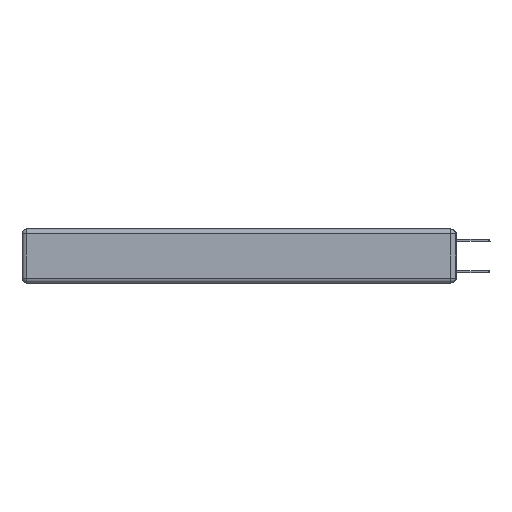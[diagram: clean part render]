
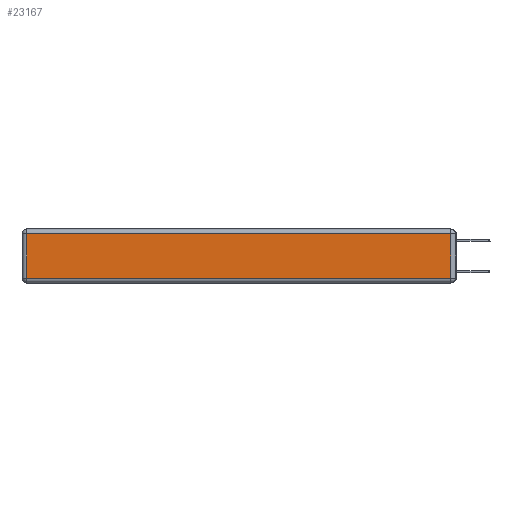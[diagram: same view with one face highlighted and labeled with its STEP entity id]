
A CAD part, left-side view. The second image highlights one B-rep face of the part: STEP entity #23167.
In plain terms, the highlighted planar face has unit normal (-1, 0, 0).
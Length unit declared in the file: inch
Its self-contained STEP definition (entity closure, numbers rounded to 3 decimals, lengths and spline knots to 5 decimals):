
#309 = DIRECTION ( 'NONE',  ( 0., 1., 0. ) ) ;
#857 = EDGE_CURVE ( 'NONE', #17902, #1594, #20052, .T. ) ;
#974 = CARTESIAN_POINT ( 'NONE',  ( 0., 2.72, -0.313 ) ) ;
#1301 = EDGE_CURVE ( 'NONE', #1594, #5061, #3868, .T. ) ;
#1594 = VERTEX_POINT ( 'NONE', #21425 ) ;
#1880 = ORIENTED_EDGE ( 'NONE', *, *, #857, .T. ) ;
#2568 = VECTOR ( 'NONE', #7059, 39.37008 ) ;
#2606 = VECTOR ( 'NONE', #11007, 39.37008 ) ;
#3868 = LINE ( 'NONE', #16387, #11226 ) ;
#5061 = VERTEX_POINT ( 'NONE', #16418 ) ;
#5471 = VECTOR ( 'NONE', #5655, 39.37008 ) ;
#5655 = DIRECTION ( 'NONE',  ( 0., -1., 0. ) ) ;
#7059 = DIRECTION ( 'NONE',  ( 0., 0., 1. ) ) ;
#7180 = CARTESIAN_POINT ( 'NONE',  ( 0., 0., -0.313 ) ) ;
#7407 = LINE ( 'NONE', #7180, #5471 ) ;
#8812 = ORIENTED_EDGE ( 'NONE', *, *, #8959, .T. ) ;
#8893 = LINE ( 'NONE', #9234, #2606 ) ;
#8959 = EDGE_CURVE ( 'NONE', #5061, #10770, #8893, .T. ) ;
#9234 = CARTESIAN_POINT ( 'NONE',  ( 0., 2.72, -0.343 ) ) ;
#9873 = EDGE_LOOP ( 'NONE', ( #12461, #1880, #17489, #8812 ) ) ;
#10770 = VERTEX_POINT ( 'NONE', #974 ) ;
#11007 = DIRECTION ( 'NONE',  ( 0., 0., -1. ) ) ;
#11226 = VECTOR ( 'NONE', #309, 39.37008 ) ;
#11541 = EDGE_CURVE ( 'NONE', #10770, #17902, #7407, .T. ) ;
#12145 = PLANE ( 'NONE',  #18011 ) ;
#12461 = ORIENTED_EDGE ( 'NONE', *, *, #11541, .T. ) ;
#13771 = DIRECTION ( 'NONE',  ( 0., 0., 1. ) ) ;
#14777 = CARTESIAN_POINT ( 'NONE',  ( 0., 0.03, -0.313 ) ) ;
#15662 = FACE_OUTER_BOUND ( 'NONE', #9873, .T. ) ;
#16387 = CARTESIAN_POINT ( 'NONE',  ( 0., 2.75, -0.03 ) ) ;
#16418 = CARTESIAN_POINT ( 'NONE',  ( 0., 2.72, -0.03 ) ) ;
#17489 = ORIENTED_EDGE ( 'NONE', *, *, #1301, .T. ) ;
#17546 = CARTESIAN_POINT ( 'NONE',  ( 0., 0., -0.343 ) ) ;
#17902 = VERTEX_POINT ( 'NONE', #14777 ) ;
#18011 = AXIS2_PLACEMENT_3D ( 'NONE', #17546, #19305, #13771 ) ;
#19305 = DIRECTION ( 'NONE',  ( -1., 0., 0. ) ) ;
#20052 = LINE ( 'NONE', #23154, #2568 ) ;
#21425 = CARTESIAN_POINT ( 'NONE',  ( 0., 0.03, -0.03 ) ) ;
#23154 = CARTESIAN_POINT ( 'NONE',  ( 0., 0.03, -0.343 ) ) ;
#23167 = ADVANCED_FACE ( 'NONE', ( #15662 ), #12145, .T. ) ;
